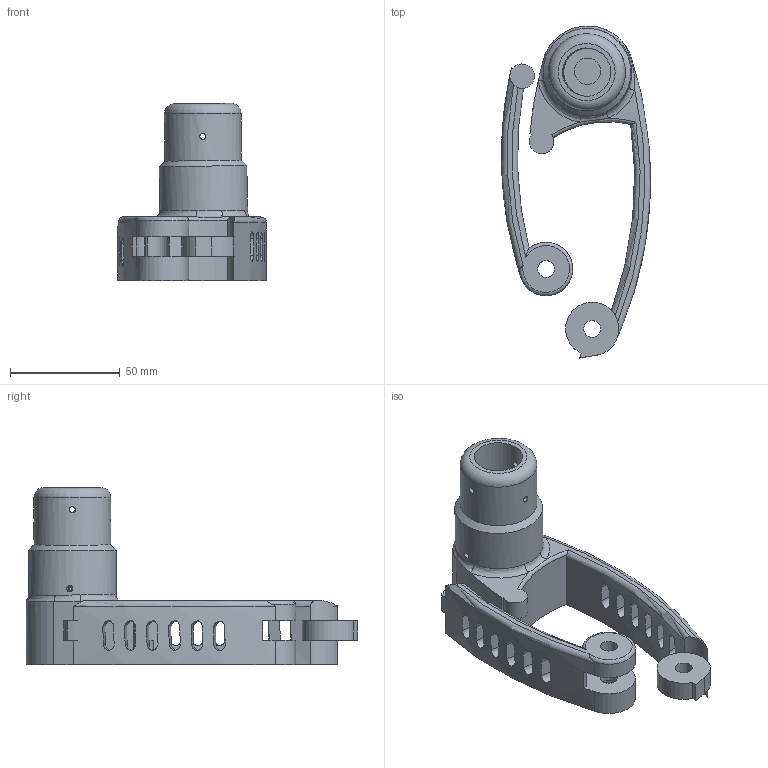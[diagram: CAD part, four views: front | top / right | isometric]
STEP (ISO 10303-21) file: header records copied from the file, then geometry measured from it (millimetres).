
FILE_DESCRIPTION(/* description */ (''),/* implementation_level */ '2;1');
FILE_NAME(/* name */ 'tailhook brace final.stp',/* time_stamp */ '2020-07-11T18:38:26-04:00',/* author */ (''),/* organization */ (''),/* preprocessor_version */ 'ST-DEVELOPER v15.2',/* originating_system */ 'Autodesk Translator Framework v2.0.0.5431',/* authorisation */ '');
FILE_SCHEMA (('AUTOMOTIVE_DESIGN { 1 0 10303 214 3 1 1 }'));
Length unit declared in the file: centimetre
Products named in the file (1): (Unsaved)
Bounding box: 67.94 x 151.37 x 80.84 mm (x, y, z)
Volume: 130800.2 mm3; surface area: 39942.4 mm2
Topology: 2 solids, 2 shells, 181 faces, 508 edges, 334 vertices
Faces by surface type: cylinder 88, plane 58, bspline 27, torus 7, cone 1
Full cylindrical faces by diameter (mm): 2.8 x7, 7.65 x3, 12 x1, 22 x2, 35 x1, 40 x1
Entity records: 16126 total; most frequent: CARTESIAN_POINT 11790, ORIENTED_EDGE 962, DIRECTION 772, EDGE_CURVE 481, VERTEX_POINT 325, AXIS2_PLACEMENT_3D 314, EDGE_LOOP 243, ADVANCED_FACE 181
